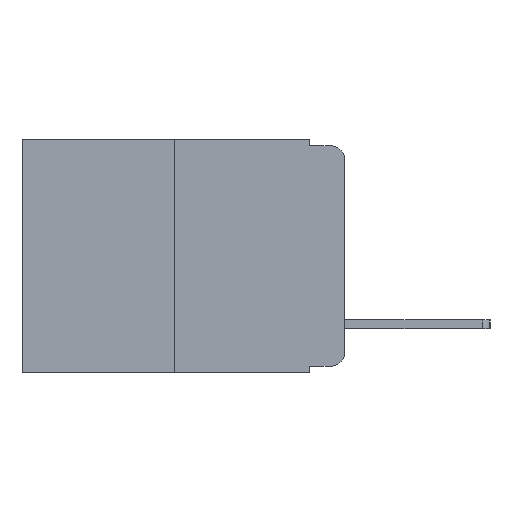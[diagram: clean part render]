
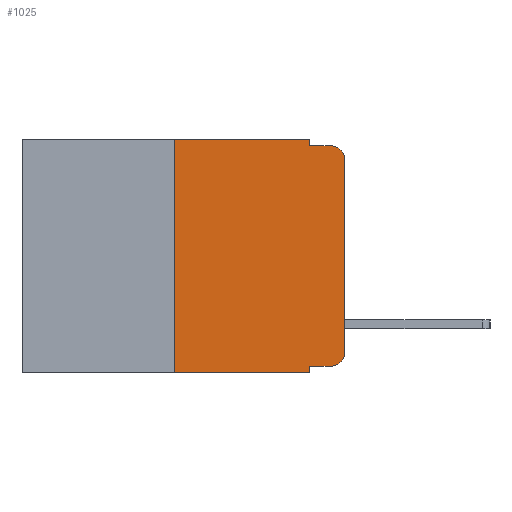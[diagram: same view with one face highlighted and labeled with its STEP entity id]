
A CAD part, left-side view. The second image highlights one B-rep face of the part: STEP entity #1025.
In plain terms, the highlighted planar face has unit normal (-1, 0, 0).
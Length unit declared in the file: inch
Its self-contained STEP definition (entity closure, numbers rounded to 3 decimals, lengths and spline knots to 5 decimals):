
#245 = LINE ( 'NONE', #10468, #4962 ) ;
#248 = DIRECTION ( 'NONE',  ( 0., 0., -1. ) ) ;
#294 = PLANE ( 'NONE',  #4498 ) ;
#370 = LINE ( 'NONE', #11199, #4503 ) ;
#690 = DIRECTION ( 'NONE',  ( 0., 0., -1. ) ) ;
#710 = DIRECTION ( 'NONE',  ( 0., 0., -1. ) ) ;
#1025 = ADVANCED_FACE ( 'NONE', ( #1865 ), #294, .F. ) ;
#1110 = ORIENTED_EDGE ( 'NONE', *, *, #7376, .F. ) ;
#1394 = ORIENTED_EDGE ( 'NONE', *, *, #2304, .F. ) ;
#1487 = CIRCLE ( 'NONE', #1659, 0.02 ) ;
#1570 = CARTESIAN_POINT ( 'NONE',  ( 0., 0.051, 0. ) ) ;
#1609 = VECTOR ( 'NONE', #7075, 39.37008 ) ;
#1659 = AXIS2_PLACEMENT_3D ( 'NONE', #5408, #5892, #3955 ) ;
#1692 = LINE ( 'NONE', #11393, #4192 ) ;
#1740 = EDGE_LOOP ( 'NONE', ( #7967, #10269, #1110, #1394, #10789, #6473, #11051, #4445, #4724, #4997 ) ) ;
#1865 = FACE_OUTER_BOUND ( 'NONE', #1740, .T. ) ;
#2146 = CIRCLE ( 'NONE', #9022, 0.02 ) ;
#2304 = EDGE_CURVE ( 'NONE', #2527, #4623, #9614, .T. ) ;
#2527 = VERTEX_POINT ( 'NONE', #1570 ) ;
#2958 = VERTEX_POINT ( 'NONE', #5347 ) ;
#3275 = CARTESIAN_POINT ( 'NONE',  ( 0., 0.473, -0.343 ) ) ;
#3406 = DIRECTION ( 'NONE',  ( 0., -1., 0. ) ) ;
#3628 = LINE ( 'NONE', #3275, #7959 ) ;
#3766 = EDGE_CURVE ( 'NONE', #6996, #2958, #245, .T. ) ;
#3955 = DIRECTION ( 'NONE',  ( 0., 0., -1. ) ) ;
#4180 = DIRECTION ( 'NONE',  ( 1., 0., 0. ) ) ;
#4185 = CARTESIAN_POINT ( 'NONE',  ( 0., 0.473, 0. ) ) ;
#4192 = VECTOR ( 'NONE', #4505, 39.37008 ) ;
#4288 = CARTESIAN_POINT ( 'NONE',  ( 0., 0., -0.313 ) ) ;
#4445 = ORIENTED_EDGE ( 'NONE', *, *, #6667, .F. ) ;
#4492 = DIRECTION ( 'NONE',  ( 0., -1., 0. ) ) ;
#4498 = AXIS2_PLACEMENT_3D ( 'NONE', #4185, #4180, #690 ) ;
#4503 = VECTOR ( 'NONE', #4492, 39.37008 ) ;
#4505 = DIRECTION ( 'NONE',  ( 0., -1., 0. ) ) ;
#4616 = CARTESIAN_POINT ( 'NONE',  ( 0., 0.051, -0.01 ) ) ;
#4623 = VERTEX_POINT ( 'NONE', #4616 ) ;
#4724 = ORIENTED_EDGE ( 'NONE', *, *, #4939, .T. ) ;
#4783 = CARTESIAN_POINT ( 'NONE',  ( 0., 0.051, -0.343 ) ) ;
#4939 = EDGE_CURVE ( 'NONE', #10585, #10910, #7073, .T. ) ;
#4962 = VECTOR ( 'NONE', #10458, 39.37008 ) ;
#4992 = VECTOR ( 'NONE', #248, 39.37008 ) ;
#4997 = ORIENTED_EDGE ( 'NONE', *, *, #6076, .T. ) ;
#5330 = DIRECTION ( 'NONE',  ( 0., 0., 1. ) ) ;
#5347 = CARTESIAN_POINT ( 'NONE',  ( 0., 0.25, 0. ) ) ;
#5408 = CARTESIAN_POINT ( 'NONE',  ( 0., 0.02, -0.313 ) ) ;
#5892 = DIRECTION ( 'NONE',  ( -1., 0., 0. ) ) ;
#6076 = EDGE_CURVE ( 'NONE', #10910, #8158, #1487, .T. ) ;
#6156 = DIRECTION ( 'NONE',  ( -1., 0., 0. ) ) ;
#6473 = ORIENTED_EDGE ( 'NONE', *, *, #3766, .F. ) ;
#6514 = VERTEX_POINT ( 'NONE', #9900 ) ;
#6667 = EDGE_CURVE ( 'NONE', #10585, #10452, #10997, .T. ) ;
#6670 = VERTEX_POINT ( 'NONE', #7135 ) ;
#6996 = VERTEX_POINT ( 'NONE', #8502 ) ;
#7073 = LINE ( 'NONE', #7387, #9417 ) ;
#7075 = DIRECTION ( 'NONE',  ( 0., 0., -1. ) ) ;
#7135 = CARTESIAN_POINT ( 'NONE',  ( 0., 0., -0.03 ) ) ;
#7163 = CARTESIAN_POINT ( 'NONE',  ( 0., 0.051, 0. ) ) ;
#7376 = EDGE_CURVE ( 'NONE', #4623, #6514, #370, .T. ) ;
#7387 = CARTESIAN_POINT ( 'NONE',  ( 0., 0.051, -0.333 ) ) ;
#7959 = VECTOR ( 'NONE', #11063, 39.37008 ) ;
#7967 = ORIENTED_EDGE ( 'NONE', *, *, #10274, .T. ) ;
#8158 = VERTEX_POINT ( 'NONE', #4288 ) ;
#8502 = CARTESIAN_POINT ( 'NONE',  ( 0., 0.25, -0.343 ) ) ;
#9022 = AXIS2_PLACEMENT_3D ( 'NONE', #11337, #6156, #710 ) ;
#9417 = VECTOR ( 'NONE', #3406, 39.37008 ) ;
#9614 = LINE ( 'NONE', #11535, #4992 ) ;
#9708 = EDGE_CURVE ( 'NONE', #6996, #10452, #3628, .T. ) ;
#9900 = CARTESIAN_POINT ( 'NONE',  ( 0., 0.02, -0.01 ) ) ;
#10236 = EDGE_CURVE ( 'NONE', #6670, #6514, #2146, .T. ) ;
#10269 = ORIENTED_EDGE ( 'NONE', *, *, #10236, .T. ) ;
#10274 = EDGE_CURVE ( 'NONE', #8158, #6670, #11428, .T. ) ;
#10452 = VERTEX_POINT ( 'NONE', #4783 ) ;
#10458 = DIRECTION ( 'NONE',  ( 0., 0., 1. ) ) ;
#10468 = CARTESIAN_POINT ( 'NONE',  ( 0., 0.25, 0. ) ) ;
#10474 = CARTESIAN_POINT ( 'NONE',  ( 0., 0.02, -0.333 ) ) ;
#10516 = CARTESIAN_POINT ( 'NONE',  ( 0., 0., 0. ) ) ;
#10585 = VERTEX_POINT ( 'NONE', #10964 ) ;
#10789 = ORIENTED_EDGE ( 'NONE', *, *, #10948, .F. ) ;
#10905 = VECTOR ( 'NONE', #5330, 39.37008 ) ;
#10910 = VERTEX_POINT ( 'NONE', #10474 ) ;
#10948 = EDGE_CURVE ( 'NONE', #2958, #2527, #1692, .T. ) ;
#10964 = CARTESIAN_POINT ( 'NONE',  ( 0., 0.051, -0.333 ) ) ;
#10997 = LINE ( 'NONE', #7163, #1609 ) ;
#11051 = ORIENTED_EDGE ( 'NONE', *, *, #9708, .T. ) ;
#11063 = DIRECTION ( 'NONE',  ( 0., -1., 0. ) ) ;
#11199 = CARTESIAN_POINT ( 'NONE',  ( 0., 0.051, -0.01 ) ) ;
#11337 = CARTESIAN_POINT ( 'NONE',  ( 0., 0.02, -0.03 ) ) ;
#11393 = CARTESIAN_POINT ( 'NONE',  ( 0., 0.473, 0. ) ) ;
#11428 = LINE ( 'NONE', #10516, #10905 ) ;
#11535 = CARTESIAN_POINT ( 'NONE',  ( 0., 0.051, 0. ) ) ;
